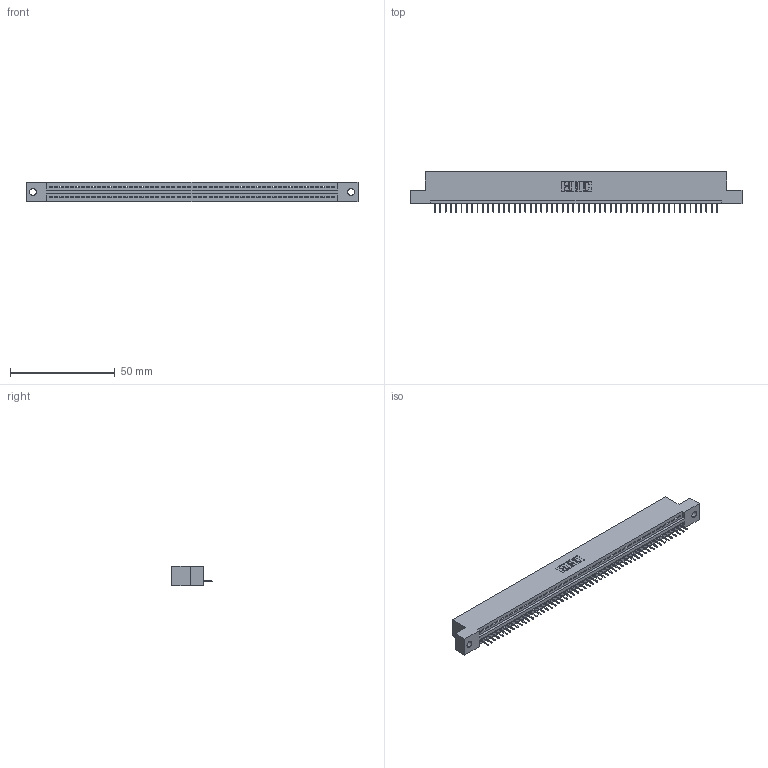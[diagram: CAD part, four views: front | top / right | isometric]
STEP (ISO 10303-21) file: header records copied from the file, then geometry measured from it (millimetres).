
FILE_DESCRIPTION (( 'STEP AP203' ), '1' );
FILE_NAME ('345-054-524-102.STEP', '2018-09-23T21:42:57', ( '' ), ( '' ), 'SwSTEP 2.0', 'SolidWorks 2016', '' );
FILE_SCHEMA (( 'CONFIG_CONTROL_DESIGN' ));
Length unit declared in the file: inch
Products named in the file (3): 345 Part_Flush Mounting Lugs - 0.128 Dia; 345-292-001_345-293-124; 345-054-524-102
Assembly tree (55 placements, depth 2):
  345-054-524-102
    345 Part_Flush Mounting Lugs - 0.128 Dia
    345-292-001_345-293-124  x54
Bounding box: 158.37 x 19.35 x 9.4 mm (x, y, z)
Volume: 14890.4 mm3; surface area: 18997.5 mm2
Topology: 55 solids, 55 shells, 3474 faces, 10061 edges, 6490 vertices
Faces by surface type: plane 2564, cylinder 910
Entity records: 39103 total; most frequent: CARTESIAN_POINT 6778, ORIENTED_EDGE 6766, DIRECTION 5903, EDGE_CURVE 3383, LINE 3039, VECTOR 3039, VERTEX_POINT 2250, AXIS2_PLACEMENT_3D 1432
